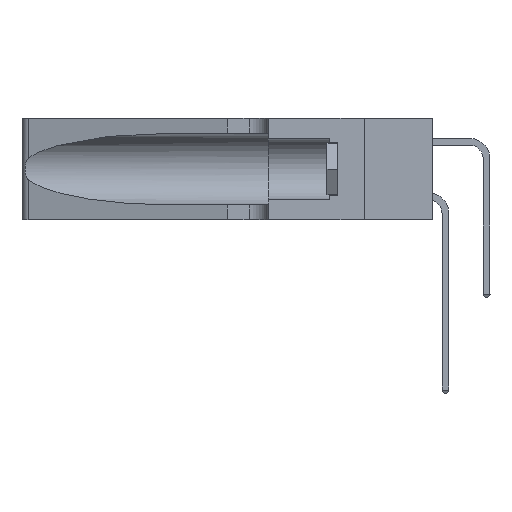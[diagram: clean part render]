
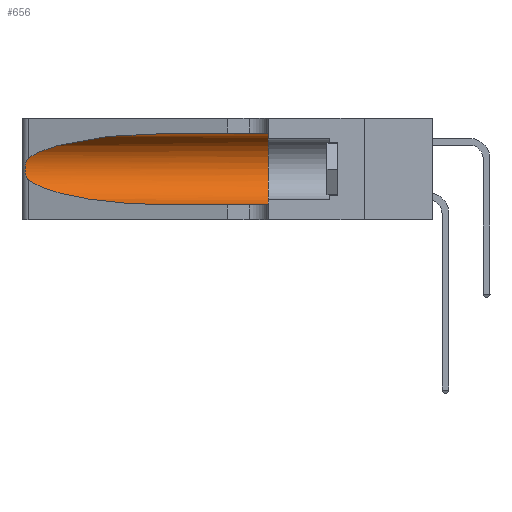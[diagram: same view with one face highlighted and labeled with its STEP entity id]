
A CAD part, left-side view. The second image highlights one B-rep face of the part: STEP entity #656.
In plain terms, the highlighted cylindrical face has radius 3.308 mm (diameter 6.617 mm), a partial arc.
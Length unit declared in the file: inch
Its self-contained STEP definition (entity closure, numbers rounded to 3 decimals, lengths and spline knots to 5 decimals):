
#313 = VERTEX_POINT ( 'NONE', #6216 ) ;
#576 = CARTESIAN_POINT ( 'NONE',  ( 0.25639, 1.23186, 0.15144 ) ) ;
#656 = ADVANCED_FACE ( 'NONE', ( #2233 ), #3377, .F. ) ;
#733 =( BOUNDED_CURVE ( )  B_SPLINE_CURVE ( 3, ( #11594, #14572, #2452, #14892 ),
 .UNSPECIFIED., .F., .F. ) 
 B_SPLINE_CURVE_WITH_KNOTS ( ( 4, 4 ),
 ( 1.5708, 2.84003 ),
 .UNSPECIFIED. ) 
 CURVE ( )  GEOMETRIC_REPRESENTATION_ITEM ( )  RATIONAL_B_SPLINE_CURVE ( ( 1., 0.87, 0.87, 1. ) ) 
 REPRESENTATION_ITEM ( '' )  );
#770 = CARTESIAN_POINT ( 'NONE',  ( 0.26017, 1.23833, 0.17102 ) ) ;
#895 = ORIENTED_EDGE ( 'NONE', *, *, #18207, .T. ) ;
#1088 = ORIENTED_EDGE ( 'NONE', *, *, #12660, .T. ) ;
#1834 = CARTESIAN_POINT ( 'NONE',  ( 0.1305, 0.72297, 0.31525 ) ) ;
#1985 = DIRECTION ( 'NONE',  ( 0., 0., 1. ) ) ;
#2233 = FACE_OUTER_BOUND ( 'NONE', #7901, .T. ) ;
#2452 = CARTESIAN_POINT ( 'NONE',  ( 0.2373, 1.15595, 0.28018 ) ) ;
#2989 = CARTESIAN_POINT ( 'NONE',  ( 0.1305, 1.61858, 0.05475 ) ) ;
#3377 = CYLINDRICAL_SURFACE ( 'NONE', #17494, 0.13025 ) ;
#4436 = CARTESIAN_POINT ( 'NONE',  ( 0.18966, 0.96281, 0.05475 ) ) ;
#4734 =( BOUNDED_CURVE ( )  B_SPLINE_CURVE ( 3, ( #17895, #6076, #4436, #7564 ),
 .UNSPECIFIED., .F., .T. ) 
 B_SPLINE_CURVE_WITH_KNOTS ( ( 4, 4 ),
 ( 3.44316, 4.71239 ),
 .UNSPECIFIED. ) 
 CURVE ( )  GEOMETRIC_REPRESENTATION_ITEM ( )  RATIONAL_B_SPLINE_CURVE ( ( 1., 0.87, 0.87, 1. ) ) 
 REPRESENTATION_ITEM ( '' )  );
#5076 = VERTEX_POINT ( 'NONE', #15960 ) ;
#5099 = CARTESIAN_POINT ( 'NONE',  ( 0.25639, 1.23184, 0.21858 ) ) ;
#5865 = CARTESIAN_POINT ( 'NONE',  ( 0.25487, 1.22718, 0.14631 ) ) ;
#6076 = CARTESIAN_POINT ( 'NONE',  ( 0.2373, 1.15595, 0.08982 ) ) ;
#6077 = EDGE_CURVE ( 'NONE', #9777, #10336, #12482, .T. ) ;
#6216 = CARTESIAN_POINT ( 'NONE',  ( 0.1305, 0.72297, 0.05475 ) ) ;
#6299 = ORIENTED_EDGE ( 'NONE', *, *, #14576, .T. ) ;
#6608 = CARTESIAN_POINT ( 'NONE',  ( 0.25555, 1.22993, 0.14849 ) ) ;
#6737 = CARTESIAN_POINT ( 'NONE',  ( 0.26018, 1.23835, 0.19895 ) ) ;
#6898 = CARTESIAN_POINT ( 'NONE',  ( 0.1305, 0.35, 0.05475 ) ) ;
#7564 = CARTESIAN_POINT ( 'NONE',  ( 0.1305, 0.72297, 0.05475 ) ) ;
#7901 = EDGE_LOOP ( 'NONE', ( #6299, #18538, #1088, #895, #10481, #9315 ) ) ;
#8063 = VECTOR ( 'NONE', #14072, 39.37008 ) ;
#8154 = CARTESIAN_POINT ( 'NONE',  ( 0.25854, 1.2359, 0.20912 ) ) ;
#8375 = EDGE_CURVE ( 'NONE', #10336, #13830, #17278, .T. ) ;
#9277 = CARTESIAN_POINT ( 'NONE',  ( 0.1305, 0.35, 0.31525 ) ) ;
#9315 = ORIENTED_EDGE ( 'NONE', *, *, #6077, .F. ) ;
#9410 = B_SPLINE_CURVE_WITH_KNOTS ( 'NONE', 3,
 ( #12515, #14018, #5099, #15630, #8154, #6737, #15496, #9671, #770, #18623, #11173, #576, #6608, #9742 ),
 .UNSPECIFIED., .F., .F.,
 ( 4, 2, 2, 2, 2, 2, 4 ),
 ( 0., 0.00027, 0.00053, 0.00107, 0.0016, 0.00187, 0.00214 ),
 .UNSPECIFIED. ) ;
#9671 = CARTESIAN_POINT ( 'NONE',  ( 0.26075, 1.23896, 0.178 ) ) ;
#9735 = CARTESIAN_POINT ( 'NONE',  ( 0.1305, 1.61858, 0.31525 ) ) ;
#9742 = CARTESIAN_POINT ( 'NONE',  ( 0.25487, 1.22718, 0.14631 ) ) ;
#9777 = VERTEX_POINT ( 'NONE', #1834 ) ;
#10233 = DIRECTION ( 'NONE',  ( 0., 0., -1. ) ) ;
#10336 = VERTEX_POINT ( 'NONE', #9277 ) ;
#10481 = ORIENTED_EDGE ( 'NONE', *, *, #8375, .F. ) ;
#11173 = CARTESIAN_POINT ( 'NONE',  ( 0.25789, 1.23486, 0.15765 ) ) ;
#11594 = CARTESIAN_POINT ( 'NONE',  ( 0.1305, 0.72297, 0.31525 ) ) ;
#12482 = LINE ( 'NONE', #9735, #8063 ) ;
#12515 = CARTESIAN_POINT ( 'NONE',  ( 0.25487, 1.22718, 0.22369 ) ) ;
#12660 = EDGE_CURVE ( 'NONE', #17691, #313, #4734, .T. ) ;
#12902 = CARTESIAN_POINT ( 'NONE',  ( 0.1305, 1.61858, 0.185 ) ) ;
#13830 = VERTEX_POINT ( 'NONE', #6898 ) ;
#14018 = CARTESIAN_POINT ( 'NONE',  ( 0.25555, 1.22994, 0.2215 ) ) ;
#14072 = DIRECTION ( 'NONE',  ( 0., -1., 0. ) ) ;
#14572 = CARTESIAN_POINT ( 'NONE',  ( 0.18966, 0.96281, 0.31525 ) ) ;
#14576 = EDGE_CURVE ( 'NONE', #9777, #5076, #733, .T. ) ;
#14703 = VECTOR ( 'NONE', #19154, 39.37008 ) ;
#14892 = CARTESIAN_POINT ( 'NONE',  ( 0.25487, 1.22718, 0.22369 ) ) ;
#15496 = CARTESIAN_POINT ( 'NONE',  ( 0.26075, 1.23896, 0.19203 ) ) ;
#15630 = CARTESIAN_POINT ( 'NONE',  ( 0.25787, 1.23484, 0.2124 ) ) ;
#15960 = CARTESIAN_POINT ( 'NONE',  ( 0.25487, 1.22718, 0.22369 ) ) ;
#16244 = EDGE_CURVE ( 'NONE', #5076, #17691, #9410, .T. ) ;
#16567 = CARTESIAN_POINT ( 'NONE',  ( 0.1305, 0.35, 0.185 ) ) ;
#16777 = DIRECTION ( 'NONE',  ( 0., 1., 0. ) ) ;
#16808 = LINE ( 'NONE', #2989, #14703 ) ;
#17060 = DIRECTION ( 'NONE',  ( 0., -1., 0. ) ) ;
#17178 = AXIS2_PLACEMENT_3D ( 'NONE', #16567, #16777, #1985 ) ;
#17278 = CIRCLE ( 'NONE', #17178, 0.13025 ) ;
#17494 = AXIS2_PLACEMENT_3D ( 'NONE', #12902, #17060, #10233 ) ;
#17691 = VERTEX_POINT ( 'NONE', #5865 ) ;
#17895 = CARTESIAN_POINT ( 'NONE',  ( 0.25487, 1.22718, 0.14631 ) ) ;
#18207 = EDGE_CURVE ( 'NONE', #313, #13830, #16808, .T. ) ;
#18538 = ORIENTED_EDGE ( 'NONE', *, *, #16244, .T. ) ;
#18623 = CARTESIAN_POINT ( 'NONE',  ( 0.25856, 1.23593, 0.16098 ) ) ;
#19154 = DIRECTION ( 'NONE',  ( 0., -1., 0. ) ) ;
